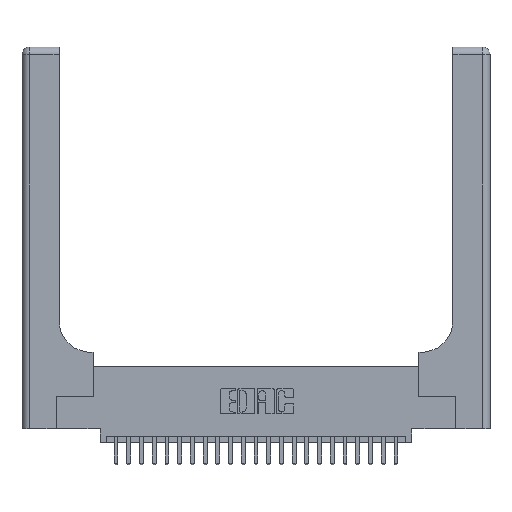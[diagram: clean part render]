
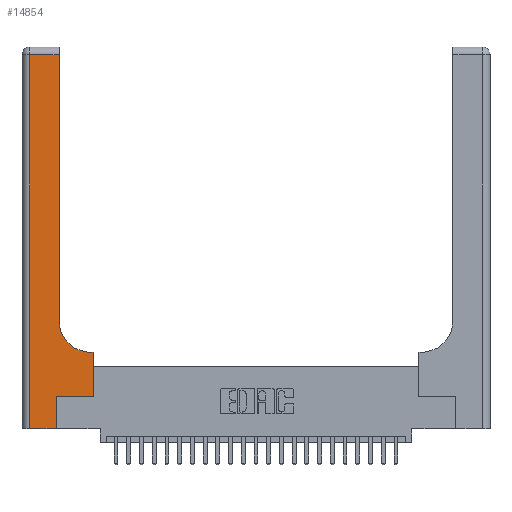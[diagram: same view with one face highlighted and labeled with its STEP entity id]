
A CAD part, top view. The second image highlights one B-rep face of the part: STEP entity #14854.
In plain terms, the highlighted planar face has unit normal (0, 0, 1).
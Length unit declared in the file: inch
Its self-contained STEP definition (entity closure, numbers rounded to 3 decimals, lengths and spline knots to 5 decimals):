
#138 = VECTOR ( 'NONE', #6675, 39.37008 ) ;
#982 = CIRCLE ( 'NONE', #8710, 0.25 ) ;
#1052 = DIRECTION ( 'NONE',  ( 1., 0., 0. ) ) ;
#1393 = CARTESIAN_POINT ( 'NONE',  ( 0.5585, 0.25, 0.37 ) ) ;
#1448 = CARTESIAN_POINT ( 'NONE',  ( 0.06, 0., 0.37 ) ) ;
#2308 = VECTOR ( 'NONE', #15682, 39.37008 ) ;
#2335 = ORIENTED_EDGE ( 'NONE', *, *, #25927, .T. ) ;
#2361 = CARTESIAN_POINT ( 'NONE',  ( 0.269, 0.25, 0.37 ) ) ;
#3086 = EDGE_LOOP ( 'NONE', ( #2335, #16847, #25128, #23604, #4789, #14949, #11403, #25861, #13384 ) ) ;
#3100 = DIRECTION ( 'NONE',  ( 0., 1., 0. ) ) ;
#3437 = VECTOR ( 'NONE', #3100, 39.37008 ) ;
#3867 = VECTOR ( 'NONE', #16811, 39.37008 ) ;
#4593 = CARTESIAN_POINT ( 'NONE',  ( 0.2915, 0.6, 0.37 ) ) ;
#4679 = CARTESIAN_POINT ( 'NONE',  ( 0., 2.94, 0.37 ) ) ;
#4693 = EDGE_CURVE ( 'NONE', #20879, #23802, #982, .T. ) ;
#4789 = ORIENTED_EDGE ( 'NONE', *, *, #11463, .T. ) ;
#4856 = DIRECTION ( 'NONE',  ( 0., 0., -1. ) ) ;
#4894 = LINE ( 'NONE', #2361, #24882 ) ;
#5965 = VERTEX_POINT ( 'NONE', #11117 ) ;
#6216 = VERTEX_POINT ( 'NONE', #13914 ) ;
#6359 = LINE ( 'NONE', #14075, #16470 ) ;
#6527 = DIRECTION ( 'NONE',  ( 1., 0., 0. ) ) ;
#6675 = DIRECTION ( 'NONE',  ( -1., 0., 0. ) ) ;
#7433 = VECTOR ( 'NONE', #11695, 39.37008 ) ;
#7482 = FACE_OUTER_BOUND ( 'NONE', #3086, .T. ) ;
#8048 = LINE ( 'NONE', #1393, #7433 ) ;
#8710 = AXIS2_PLACEMENT_3D ( 'NONE', #25121, #13383, #1052 ) ;
#9333 = EDGE_CURVE ( 'NONE', #5965, #21800, #8048, .T. ) ;
#9349 = LINE ( 'NONE', #4679, #3867 ) ;
#10523 = VERTEX_POINT ( 'NONE', #16623 ) ;
#11117 = CARTESIAN_POINT ( 'NONE',  ( 0.5585, 0.25, 0.37 ) ) ;
#11403 = ORIENTED_EDGE ( 'NONE', *, *, #9333, .T. ) ;
#11463 = EDGE_CURVE ( 'NONE', #6216, #10523, #25341, .T. ) ;
#11695 = DIRECTION ( 'NONE',  ( 0., 1., 0. ) ) ;
#11822 = LINE ( 'NONE', #4593, #138 ) ;
#11855 = VECTOR ( 'NONE', #24721, 39.37008 ) ;
#13383 = DIRECTION ( 'NONE',  ( 0., 0., -1. ) ) ;
#13384 = ORIENTED_EDGE ( 'NONE', *, *, #4693, .T. ) ;
#13390 = CARTESIAN_POINT ( 'NONE',  ( 0.5585, 0.6, 0.37 ) ) ;
#13686 = CARTESIAN_POINT ( 'NONE',  ( 0.06, 3., 0.37 ) ) ;
#13914 = CARTESIAN_POINT ( 'NONE',  ( 0.269, 0., 0.37 ) ) ;
#14075 = CARTESIAN_POINT ( 'NONE',  ( 0., 0., 0.37 ) ) ;
#14854 = ADVANCED_FACE ( 'NONE', ( #7482 ), #16881, .F. ) ;
#14949 = ORIENTED_EDGE ( 'NONE', *, *, #22821, .T. ) ;
#15311 = AXIS2_PLACEMENT_3D ( 'NONE', #16961, #4856, #18921 ) ;
#15682 = DIRECTION ( 'NONE',  ( 0., -1., 0. ) ) ;
#16058 = DIRECTION ( 'NONE',  ( 1., 0., 0. ) ) ;
#16470 = VECTOR ( 'NONE', #16058, 39.37008 ) ;
#16542 = VERTEX_POINT ( 'NONE', #20141 ) ;
#16623 = CARTESIAN_POINT ( 'NONE',  ( 0.269, 0.25, 0.37 ) ) ;
#16811 = DIRECTION ( 'NONE',  ( -1., 0., 0. ) ) ;
#16847 = ORIENTED_EDGE ( 'NONE', *, *, #24605, .T. ) ;
#16881 = PLANE ( 'NONE',  #15311 ) ;
#16961 = CARTESIAN_POINT ( 'NONE',  ( 0., 3., 0.37 ) ) ;
#18188 = EDGE_CURVE ( 'NONE', #19750, #6216, #6359, .T. ) ;
#18453 = LINE ( 'NONE', #13686, #2308 ) ;
#18921 = DIRECTION ( 'NONE',  ( -1., 0., 0. ) ) ;
#19750 = VERTEX_POINT ( 'NONE', #1448 ) ;
#20033 = EDGE_CURVE ( 'NONE', #21800, #20879, #11822, .T. ) ;
#20141 = CARTESIAN_POINT ( 'NONE',  ( 0.06, 2.94, 0.37 ) ) ;
#20879 = VERTEX_POINT ( 'NONE', #25326 ) ;
#21800 = VERTEX_POINT ( 'NONE', #13390 ) ;
#22481 = EDGE_CURVE ( 'NONE', #16542, #19750, #18453, .T. ) ;
#22768 = CARTESIAN_POINT ( 'NONE',  ( 0.2915, 3., 0.37 ) ) ;
#22821 = EDGE_CURVE ( 'NONE', #10523, #5965, #4894, .T. ) ;
#22917 = VERTEX_POINT ( 'NONE', #24725 ) ;
#23189 = CARTESIAN_POINT ( 'NONE',  ( 0.269, 0., 0.37 ) ) ;
#23604 = ORIENTED_EDGE ( 'NONE', *, *, #18188, .T. ) ;
#23802 = VERTEX_POINT ( 'NONE', #25550 ) ;
#24605 = EDGE_CURVE ( 'NONE', #22917, #16542, #9349, .T. ) ;
#24721 = DIRECTION ( 'NONE',  ( 0., 1., 0. ) ) ;
#24725 = CARTESIAN_POINT ( 'NONE',  ( 0.2915, 2.94, 0.37 ) ) ;
#24882 = VECTOR ( 'NONE', #6527, 39.37008 ) ;
#25121 = CARTESIAN_POINT ( 'NONE',  ( 0.5415, 0.85, 0.37 ) ) ;
#25128 = ORIENTED_EDGE ( 'NONE', *, *, #22481, .T. ) ;
#25326 = CARTESIAN_POINT ( 'NONE',  ( 0.5415, 0.6, 0.37 ) ) ;
#25341 = LINE ( 'NONE', #23189, #3437 ) ;
#25550 = CARTESIAN_POINT ( 'NONE',  ( 0.2915, 0.85, 0.37 ) ) ;
#25677 = LINE ( 'NONE', #22768, #11855 ) ;
#25861 = ORIENTED_EDGE ( 'NONE', *, *, #20033, .T. ) ;
#25927 = EDGE_CURVE ( 'NONE', #23802, #22917, #25677, .T. ) ;
